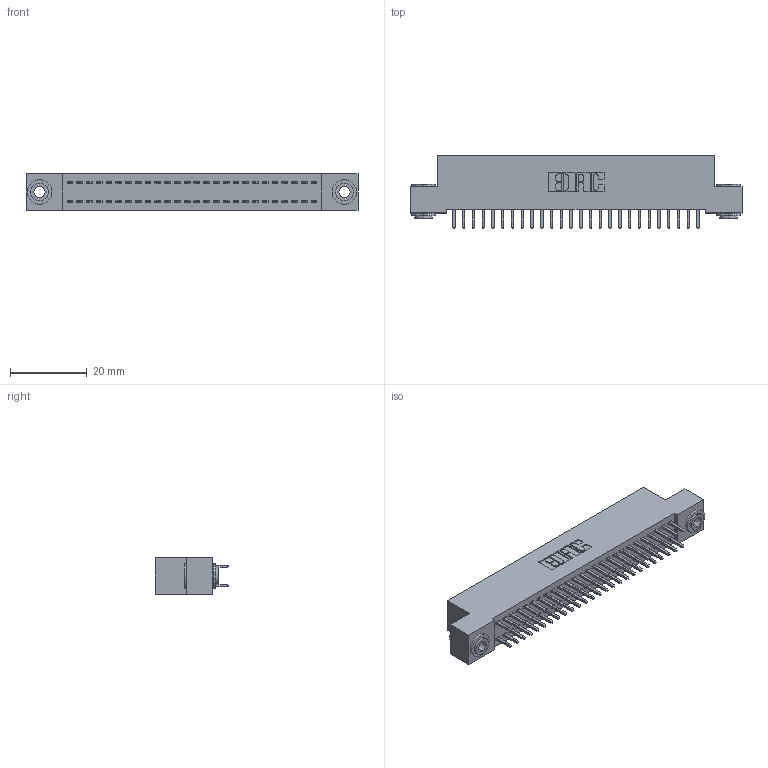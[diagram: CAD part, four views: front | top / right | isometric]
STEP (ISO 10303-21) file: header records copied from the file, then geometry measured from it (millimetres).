
FILE_DESCRIPTION (( 'STEP AP203' ), '1' );
FILE_NAME ('392-052-521-203.STEP', '2018-08-17T04:41:04', ( '' ), ( '' ), 'SwSTEP 2.0', 'SolidWorks 2016', '' );
FILE_SCHEMA (( 'CONFIG_CONTROL_DESIGN' ));
Length unit declared in the file: inch
Products named in the file (4): 392-052-521-203; 342 Part_.156 TH; 345-292-001_345-293-121; 342-250-002_345-250-002-102
Assembly tree (55 placements, depth 2):
  392-052-521-203
    342 Part_.156 TH
    345-292-001_345-293-121  x52
    342-250-002_345-250-002-102  x2
Bounding box: 86.36 x 19.06 x 9.4 mm (x, y, z)
Volume: 7685.3 mm3; surface area: 12185.9 mm2
Topology: 55 solids, 55 shells, 2852 faces, 8435 edges, 5550 vertices
Faces by surface type: plane 1948, cylinder 896, cone 8
Entity records: 19332 total; most frequent: CARTESIAN_POINT 3197, ORIENTED_EDGE 3126, DIRECTION 2793, EDGE_CURVE 1563, LINE 1411, VECTOR 1411, VERTEX_POINT 1038, AXIS2_PLACEMENT_3D 691
